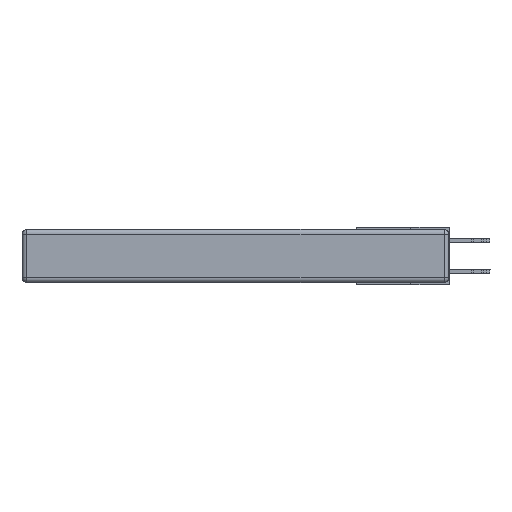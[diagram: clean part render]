
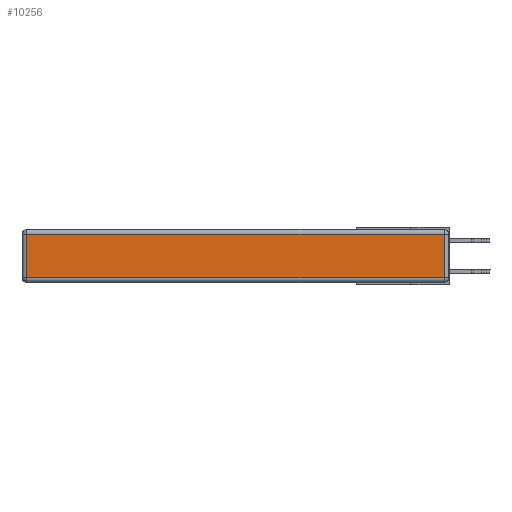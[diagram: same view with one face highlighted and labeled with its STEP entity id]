
A CAD part, left-side view. The second image highlights one B-rep face of the part: STEP entity #10256.
In plain terms, the highlighted planar face has unit normal (-1, 0, 0).
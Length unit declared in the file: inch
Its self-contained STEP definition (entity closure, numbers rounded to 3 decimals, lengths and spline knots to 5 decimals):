
#235 = CARTESIAN_POINT ( 'NONE',  ( 0., 0., -0.343 ) ) ;
#485 = ORIENTED_EDGE ( 'NONE', *, *, #9522, .T. ) ;
#495 = DIRECTION ( 'NONE',  ( 0., 0., 1. ) ) ;
#1433 = ORIENTED_EDGE ( 'NONE', *, *, #13822, .T. ) ;
#7127 = DIRECTION ( 'NONE',  ( 0., 0., 1. ) ) ;
#7537 = CARTESIAN_POINT ( 'NONE',  ( 0., 2.75, -0.03 ) ) ;
#9522 = EDGE_CURVE ( 'NONE', #34476, #18897, #11650, .T. ) ;
#10133 = CARTESIAN_POINT ( 'NONE',  ( 0., 2.72, -0.03 ) ) ;
#10256 = ADVANCED_FACE ( 'NONE', ( #32038 ), #32844, .T. ) ;
#11650 = LINE ( 'NONE', #34184, #28304 ) ;
#12109 = EDGE_CURVE ( 'NONE', #18449, #34476, #26003, .T. ) ;
#12630 = EDGE_CURVE ( 'NONE', #34911, #18449, #26360, .T. ) ;
#13822 = EDGE_CURVE ( 'NONE', #18897, #34911, #21584, .T. ) ;
#18449 = VERTEX_POINT ( 'NONE', #21514 ) ;
#18897 = VERTEX_POINT ( 'NONE', #25820 ) ;
#19108 = VECTOR ( 'NONE', #23585, 39.37008 ) ;
#19947 = VECTOR ( 'NONE', #33624, 39.37008 ) ;
#21514 = CARTESIAN_POINT ( 'NONE',  ( 0., 2.72, -0.313 ) ) ;
#21584 = LINE ( 'NONE', #7537, #22434 ) ;
#22274 = DIRECTION ( 'NONE',  ( -1., 0., 0. ) ) ;
#22434 = VECTOR ( 'NONE', #29108, 39.37008 ) ;
#23319 = CARTESIAN_POINT ( 'NONE',  ( 0., 0.03, -0.313 ) ) ;
#23585 = DIRECTION ( 'NONE',  ( 0., -1., 0. ) ) ;
#23706 = EDGE_LOOP ( 'NONE', ( #31272, #485, #1433, #34565 ) ) ;
#25170 = CARTESIAN_POINT ( 'NONE',  ( 0., 0., -0.313 ) ) ;
#25820 = CARTESIAN_POINT ( 'NONE',  ( 0., 0.03, -0.03 ) ) ;
#26003 = LINE ( 'NONE', #25170, #19108 ) ;
#26360 = LINE ( 'NONE', #30807, #19947 ) ;
#28304 = VECTOR ( 'NONE', #7127, 39.37008 ) ;
#29108 = DIRECTION ( 'NONE',  ( 0., 1., 0. ) ) ;
#30807 = CARTESIAN_POINT ( 'NONE',  ( 0., 2.72, -0.343 ) ) ;
#31272 = ORIENTED_EDGE ( 'NONE', *, *, #12109, .T. ) ;
#32038 = FACE_OUTER_BOUND ( 'NONE', #23706, .T. ) ;
#32326 = AXIS2_PLACEMENT_3D ( 'NONE', #235, #22274, #495 ) ;
#32844 = PLANE ( 'NONE',  #32326 ) ;
#33624 = DIRECTION ( 'NONE',  ( 0., 0., -1. ) ) ;
#34184 = CARTESIAN_POINT ( 'NONE',  ( 0., 0.03, -0.343 ) ) ;
#34476 = VERTEX_POINT ( 'NONE', #23319 ) ;
#34565 = ORIENTED_EDGE ( 'NONE', *, *, #12630, .T. ) ;
#34911 = VERTEX_POINT ( 'NONE', #10133 ) ;
